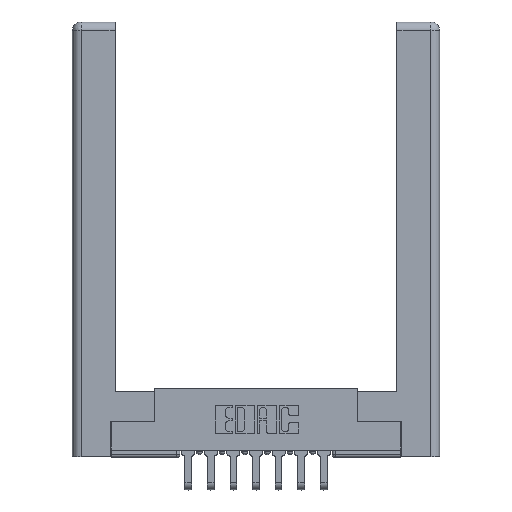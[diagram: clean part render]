
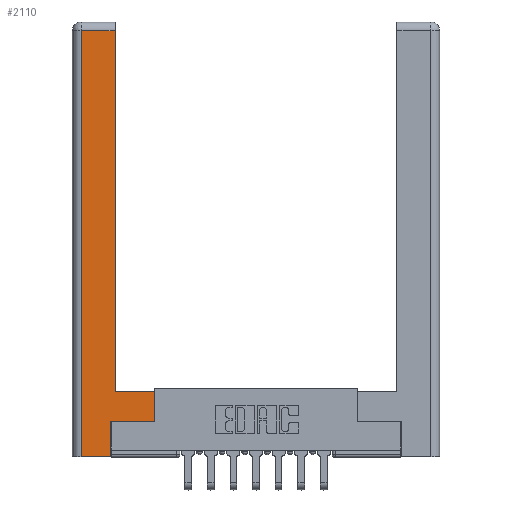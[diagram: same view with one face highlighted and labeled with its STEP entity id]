
A CAD part, top view. The second image highlights one B-rep face of the part: STEP entity #2110.
In plain terms, the highlighted planar face has unit normal (0, 0, 1).
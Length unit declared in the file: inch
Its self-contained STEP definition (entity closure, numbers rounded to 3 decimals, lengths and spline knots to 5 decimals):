
#158 = LINE ( 'NONE', #5826, #6772 ) ;
#197 = LINE ( 'NONE', #7076, #6153 ) ;
#267 = CARTESIAN_POINT ( 'NONE',  ( 0.265, 0., 0. ) ) ;
#290 = VECTOR ( 'NONE', #2038, 39.37008 ) ;
#938 = DIRECTION ( 'NONE',  ( -1., 0., 0. ) ) ;
#1084 = ORIENTED_EDGE ( 'NONE', *, *, #9360, .T. ) ;
#1285 = CARTESIAN_POINT ( 'NONE',  ( 0.265, 0.245, 0. ) ) ;
#1292 = EDGE_LOOP ( 'NONE', ( #5047, #1084, #14371, #6290, #3260, #6378, #8532, #2084 ) ) ;
#1645 = DIRECTION ( 'NONE',  ( 0., 1., 0. ) ) ;
#2038 = DIRECTION ( 'NONE',  ( -1., 0., 0. ) ) ;
#2070 = CARTESIAN_POINT ( 'NONE',  ( 0.295, 0.45, 0. ) ) ;
#2084 = ORIENTED_EDGE ( 'NONE', *, *, #5311, .T. ) ;
#2110 = ADVANCED_FACE ( 'NONE', ( #5882 ), #12737, .F. ) ;
#2184 = LINE ( 'NONE', #12216, #290 ) ;
#2383 = VERTEX_POINT ( 'NONE', #6401 ) ;
#2613 = CARTESIAN_POINT ( 'NONE',  ( 0.0615, 2.94, 0. ) ) ;
#2639 = LINE ( 'NONE', #267, #8637 ) ;
#2673 = DIRECTION ( 'NONE',  ( 0., 1., 0. ) ) ;
#2780 = VECTOR ( 'NONE', #11801, 39.37008 ) ;
#2943 = EDGE_CURVE ( 'NONE', #4631, #9813, #158, .T. ) ;
#3165 = EDGE_CURVE ( 'NONE', #12806, #2383, #6905, .T. ) ;
#3260 = ORIENTED_EDGE ( 'NONE', *, *, #5817, .T. ) ;
#3494 = CARTESIAN_POINT ( 'NONE',  ( 0.565, 0.245, 0. ) ) ;
#3667 = DIRECTION ( 'NONE',  ( 0., -1., 0. ) ) ;
#3863 = CARTESIAN_POINT ( 'NONE',  ( 0.295, 0.45, 0. ) ) ;
#4450 = VERTEX_POINT ( 'NONE', #2613 ) ;
#4631 = VERTEX_POINT ( 'NONE', #3863 ) ;
#4916 = DIRECTION ( 'NONE',  ( 0., 0., -1. ) ) ;
#5047 = ORIENTED_EDGE ( 'NONE', *, *, #2943, .T. ) ;
#5311 = EDGE_CURVE ( 'NONE', #12544, #4631, #6649, .T. ) ;
#5817 = EDGE_CURVE ( 'NONE', #7322, #12806, #10615, .T. ) ;
#5826 = CARTESIAN_POINT ( 'NONE',  ( 0.295, 3., 0. ) ) ;
#5882 = FACE_OUTER_BOUND ( 'NONE', #1292, .T. ) ;
#5938 = VECTOR ( 'NONE', #1645, 39.37008 ) ;
#6153 = VECTOR ( 'NONE', #3667, 39.37008 ) ;
#6290 = ORIENTED_EDGE ( 'NONE', *, *, #12291, .T. ) ;
#6360 = VERTEX_POINT ( 'NONE', #11948 ) ;
#6378 = ORIENTED_EDGE ( 'NONE', *, *, #3165, .T. ) ;
#6382 = VECTOR ( 'NONE', #13498, 39.37008 ) ;
#6401 = CARTESIAN_POINT ( 'NONE',  ( 0.565, 0.245, 0. ) ) ;
#6649 = LINE ( 'NONE', #2070, #10235 ) ;
#6772 = VECTOR ( 'NONE', #2673, 39.37008 ) ;
#6905 = LINE ( 'NONE', #3494, #2780 ) ;
#7076 = CARTESIAN_POINT ( 'NONE',  ( 0.0615, 0., 0. ) ) ;
#7322 = VERTEX_POINT ( 'NONE', #9321 ) ;
#7701 = CARTESIAN_POINT ( 'NONE',  ( 0.565, 0.45, 0. ) ) ;
#8532 = ORIENTED_EDGE ( 'NONE', *, *, #13060, .T. ) ;
#8637 = VECTOR ( 'NONE', #9306, 39.37008 ) ;
#8957 = LINE ( 'NONE', #7701, #6382 ) ;
#9033 = EDGE_CURVE ( 'NONE', #4450, #6360, #197, .T. ) ;
#9306 = DIRECTION ( 'NONE',  ( 1., 0., 0. ) ) ;
#9321 = CARTESIAN_POINT ( 'NONE',  ( 0.265, 0., 0. ) ) ;
#9360 = EDGE_CURVE ( 'NONE', #9813, #4450, #2184, .T. ) ;
#9813 = VERTEX_POINT ( 'NONE', #12540 ) ;
#10235 = VECTOR ( 'NONE', #938, 39.37008 ) ;
#10615 = LINE ( 'NONE', #11526, #5938 ) ;
#10641 = DIRECTION ( 'NONE',  ( -1., 0., 0. ) ) ;
#11526 = CARTESIAN_POINT ( 'NONE',  ( 0.265, 0.245, 0. ) ) ;
#11801 = DIRECTION ( 'NONE',  ( 1., 0., 0. ) ) ;
#11948 = CARTESIAN_POINT ( 'NONE',  ( 0.0615, 0., 0. ) ) ;
#12216 = CARTESIAN_POINT ( 'NONE',  ( 0.0615, 2.94, 0. ) ) ;
#12291 = EDGE_CURVE ( 'NONE', #6360, #7322, #2639, .T. ) ;
#12540 = CARTESIAN_POINT ( 'NONE',  ( 0.295, 2.94, 0. ) ) ;
#12544 = VERTEX_POINT ( 'NONE', #13309 ) ;
#12737 = PLANE ( 'NONE',  #13774 ) ;
#12806 = VERTEX_POINT ( 'NONE', #1285 ) ;
#13060 = EDGE_CURVE ( 'NONE', #2383, #12544, #8957, .T. ) ;
#13309 = CARTESIAN_POINT ( 'NONE',  ( 0.565, 0.45, 0. ) ) ;
#13498 = DIRECTION ( 'NONE',  ( 0., 1., 0. ) ) ;
#13774 = AXIS2_PLACEMENT_3D ( 'NONE', #14067, #4916, #10641 ) ;
#14067 = CARTESIAN_POINT ( 'NONE',  ( 0., 0., 0. ) ) ;
#14371 = ORIENTED_EDGE ( 'NONE', *, *, #9033, .T. ) ;
